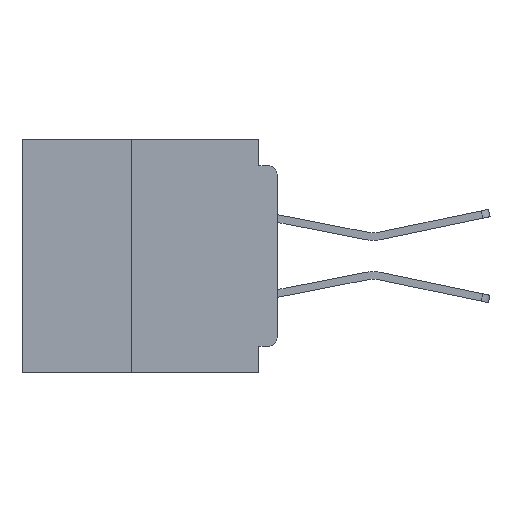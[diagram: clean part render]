
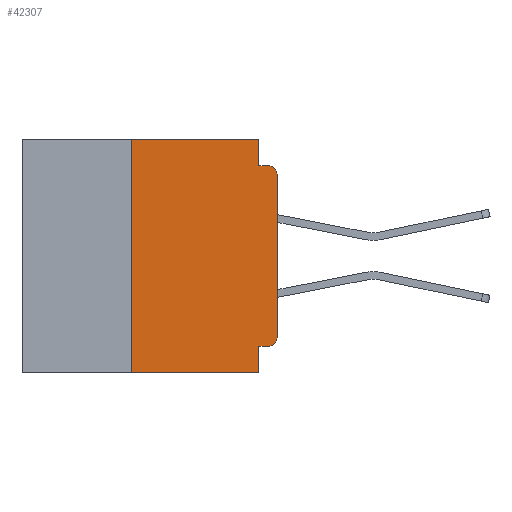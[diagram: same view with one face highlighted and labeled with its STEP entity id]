
A CAD part, left-side view. The second image highlights one B-rep face of the part: STEP entity #42307.
In plain terms, the highlighted planar face has unit normal (-1, 0, 0).
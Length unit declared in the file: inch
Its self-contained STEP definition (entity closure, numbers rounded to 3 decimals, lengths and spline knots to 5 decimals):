
#132 = FACE_OUTER_BOUND ( 'NONE', #31304, .T. ) ;
#823 = VERTEX_POINT ( 'NONE', #48053 ) ;
#2797 = EDGE_CURVE ( 'NONE', #823, #13063, #47165, .T. ) ;
#3291 = CARTESIAN_POINT ( 'NONE',  ( 0., 0.015, -0.34 ) ) ;
#3422 = EDGE_CURVE ( 'NONE', #15420, #46559, #47697, .T. ) ;
#3801 = EDGE_CURVE ( 'NONE', #24400, #15420, #29211, .T. ) ;
#4370 = ORIENTED_EDGE ( 'NONE', *, *, #3422, .F. ) ;
#6146 = EDGE_CURVE ( 'NONE', #25168, #46559, #6499, .T. ) ;
#6499 = LINE ( 'NONE', #25925, #19675 ) ;
#6562 = CARTESIAN_POINT ( 'NONE',  ( 0., 0.437, 0. ) ) ;
#7151 = VECTOR ( 'NONE', #32833, 39.37008 ) ;
#7329 = CARTESIAN_POINT ( 'NONE',  ( 0., 0.031, -0.045 ) ) ;
#7380 = DIRECTION ( 'NONE',  ( 0., 0., -1. ) ) ;
#8459 = CARTESIAN_POINT ( 'NONE',  ( 0., 0.031, 0. ) ) ;
#8597 = ORIENTED_EDGE ( 'NONE', *, *, #6146, .T. ) ;
#8873 = EDGE_CURVE ( 'NONE', #25168, #30435, #40118, .T. ) ;
#10105 = CARTESIAN_POINT ( 'NONE',  ( 0., 0.015, -0.045 ) ) ;
#10466 = CARTESIAN_POINT ( 'NONE',  ( 0., 0.015, -0.06 ) ) ;
#13063 = VERTEX_POINT ( 'NONE', #39171 ) ;
#14059 = DIRECTION ( 'NONE',  ( 1., 0., 0. ) ) ;
#14403 = VECTOR ( 'NONE', #36599, 39.37008 ) ;
#14451 = DIRECTION ( 'NONE',  ( 0., 0., -1. ) ) ;
#15314 = AXIS2_PLACEMENT_3D ( 'NONE', #10466, #38223, #14451 ) ;
#15420 = VERTEX_POINT ( 'NONE', #43957 ) ;
#18649 = VECTOR ( 'NONE', #45625, 39.37008 ) ;
#19598 = EDGE_CURVE ( 'NONE', #51324, #39305, #47286, .T. ) ;
#19675 = VECTOR ( 'NONE', #41782, 39.37008 ) ;
#22319 = CIRCLE ( 'NONE', #15314, 0.015 ) ;
#22487 = DIRECTION ( 'NONE',  ( 0., -1., 0. ) ) ;
#24040 = VECTOR ( 'NONE', #22487, 39.37008 ) ;
#24400 = VERTEX_POINT ( 'NONE', #27972 ) ;
#24686 = CARTESIAN_POINT ( 'NONE',  ( 0., 0.031, -0.4 ) ) ;
#25168 = VERTEX_POINT ( 'NONE', #48507 ) ;
#25304 = LINE ( 'NONE', #6562, #24040 ) ;
#25925 = CARTESIAN_POINT ( 'NONE',  ( 0., 0.437, -0.4 ) ) ;
#26286 = CIRCLE ( 'NONE', #40427, 0.015 ) ;
#27613 = ORIENTED_EDGE ( 'NONE', *, *, #19598, .F. ) ;
#27972 = CARTESIAN_POINT ( 'NONE',  ( 0., 0.015, -0.355 ) ) ;
#28312 = DIRECTION ( 'NONE',  ( 0., 0., -1. ) ) ;
#28434 = CARTESIAN_POINT ( 'NONE',  ( 0., 0.031, 0. ) ) ;
#28880 = CARTESIAN_POINT ( 'NONE',  ( 0., 0.25, -0.4 ) ) ;
#28983 = ORIENTED_EDGE ( 'NONE', *, *, #8873, .F. ) ;
#29211 = LINE ( 'NONE', #46270, #18649 ) ;
#29538 = ORIENTED_EDGE ( 'NONE', *, *, #3801, .F. ) ;
#29684 = VECTOR ( 'NONE', #45526, 39.37008 ) ;
#29860 = PLANE ( 'NONE',  #40276 ) ;
#30435 = VERTEX_POINT ( 'NONE', #34063 ) ;
#30514 = ORIENTED_EDGE ( 'NONE', *, *, #41796, .F. ) ;
#31237 = DIRECTION ( 'NONE',  ( -1., 0., 0. ) ) ;
#31304 = EDGE_LOOP ( 'NONE', ( #48761, #31308, #46875, #27613, #30514, #28983, #8597, #4370, #29538, #42817 ) ) ;
#31308 = ORIENTED_EDGE ( 'NONE', *, *, #49947, .T. ) ;
#31995 = CARTESIAN_POINT ( 'NONE',  ( 0., 0.031, -0.4 ) ) ;
#32833 = DIRECTION ( 'NONE',  ( 0., 0., 1. ) ) ;
#33223 = EDGE_CURVE ( 'NONE', #39305, #49918, #50536, .T. ) ;
#34063 = CARTESIAN_POINT ( 'NONE',  ( 0., 0.25, 0. ) ) ;
#34239 = DIRECTION ( 'NONE',  ( 0., 0., -1. ) ) ;
#36599 = DIRECTION ( 'NONE',  ( 0., 0., 1. ) ) ;
#36888 = EDGE_CURVE ( 'NONE', #24400, #823, #26286, .T. ) ;
#37639 = CARTESIAN_POINT ( 'NONE',  ( 0., 0., -0.045 ) ) ;
#38223 = DIRECTION ( 'NONE',  ( -1., 0., 0. ) ) ;
#38233 = CARTESIAN_POINT ( 'NONE',  ( 0., 0., 0. ) ) ;
#38540 = VECTOR ( 'NONE', #34239, 39.37008 ) ;
#39171 = CARTESIAN_POINT ( 'NONE',  ( 0., 0., -0.06 ) ) ;
#39305 = VERTEX_POINT ( 'NONE', #7329 ) ;
#40118 = LINE ( 'NONE', #28880, #7151 ) ;
#40276 = AXIS2_PLACEMENT_3D ( 'NONE', #41602, #14059, #41769 ) ;
#40427 = AXIS2_PLACEMENT_3D ( 'NONE', #3291, #31237, #7380 ) ;
#41602 = CARTESIAN_POINT ( 'NONE',  ( 0., 0.437, 0. ) ) ;
#41769 = DIRECTION ( 'NONE',  ( 0., 0., -1. ) ) ;
#41782 = DIRECTION ( 'NONE',  ( 0., -1., 0. ) ) ;
#41796 = EDGE_CURVE ( 'NONE', #30435, #51324, #25304, .T. ) ;
#42307 = ADVANCED_FACE ( 'NONE', ( #132 ), #29860, .F. ) ;
#42817 = ORIENTED_EDGE ( 'NONE', *, *, #36888, .T. ) ;
#43957 = CARTESIAN_POINT ( 'NONE',  ( 0., 0.031, -0.355 ) ) ;
#45526 = DIRECTION ( 'NONE',  ( 0., -1., 0. ) ) ;
#45625 = DIRECTION ( 'NONE',  ( 0., 1., 0. ) ) ;
#46081 = VECTOR ( 'NONE', #28312, 39.37008 ) ;
#46270 = CARTESIAN_POINT ( 'NONE',  ( 0., 0., -0.355 ) ) ;
#46559 = VERTEX_POINT ( 'NONE', #24686 ) ;
#46875 = ORIENTED_EDGE ( 'NONE', *, *, #33223, .F. ) ;
#47165 = LINE ( 'NONE', #38233, #14403 ) ;
#47286 = LINE ( 'NONE', #8459, #46081 ) ;
#47697 = LINE ( 'NONE', #31995, #38540 ) ;
#48053 = CARTESIAN_POINT ( 'NONE',  ( 0., 0., -0.34 ) ) ;
#48507 = CARTESIAN_POINT ( 'NONE',  ( 0., 0.25, -0.4 ) ) ;
#48761 = ORIENTED_EDGE ( 'NONE', *, *, #2797, .T. ) ;
#49918 = VERTEX_POINT ( 'NONE', #10105 ) ;
#49947 = EDGE_CURVE ( 'NONE', #13063, #49918, #22319, .T. ) ;
#50536 = LINE ( 'NONE', #37639, #29684 ) ;
#51324 = VERTEX_POINT ( 'NONE', #28434 ) ;
